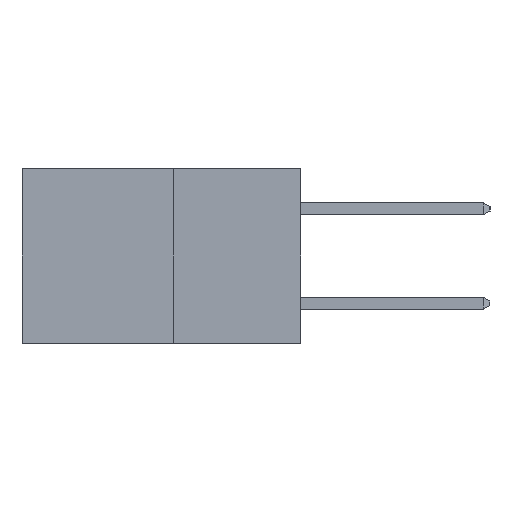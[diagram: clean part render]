
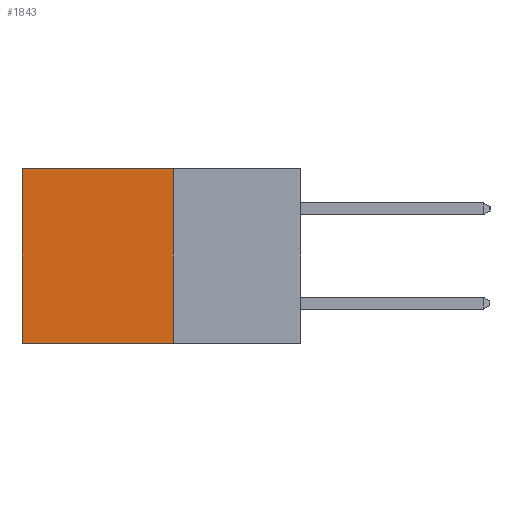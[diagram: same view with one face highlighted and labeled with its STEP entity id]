
A CAD part, left-side view. The second image highlights one B-rep face of the part: STEP entity #1843.
In plain terms, the highlighted planar face has unit normal (-1, 0, 0).
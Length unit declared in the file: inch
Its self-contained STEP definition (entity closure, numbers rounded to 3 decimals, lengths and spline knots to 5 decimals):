
#113 = ORIENTED_EDGE ( 'NONE', *, *, #7883, .F. ) ;
#327 = VERTEX_POINT ( 'NONE', #982 ) ;
#608 = CARTESIAN_POINT ( 'NONE',  ( 0.277, 0.27, 0. ) ) ;
#847 = ORIENTED_EDGE ( 'NONE', *, *, #9786, .T. ) ;
#982 = CARTESIAN_POINT ( 'NONE',  ( 0.277, 0.59, -0.37 ) ) ;
#1668 = AXIS2_PLACEMENT_3D ( 'NONE', #6906, #10502, #9858 ) ;
#1713 = DIRECTION ( 'NONE',  ( 0., 0., -1. ) ) ;
#1843 = ADVANCED_FACE ( 'NONE', ( #11647 ), #8633, .F. ) ;
#1958 = VECTOR ( 'NONE', #9533, 39.37008 ) ;
#2828 = CARTESIAN_POINT ( 'NONE',  ( 0.277, 0.27, -0.37 ) ) ;
#2880 = CARTESIAN_POINT ( 'NONE',  ( 0.277, 0.27, -0.37 ) ) ;
#4677 = DIRECTION ( 'NONE',  ( 0., 1., 0. ) ) ;
#4868 = LINE ( 'NONE', #8497, #1958 ) ;
#6008 = EDGE_CURVE ( 'NONE', #12313, #327, #11225, .T. ) ;
#6906 = CARTESIAN_POINT ( 'NONE',  ( 0.277, 0.27, -0.37 ) ) ;
#7883 = EDGE_CURVE ( 'NONE', #11270, #327, #4868, .T. ) ;
#8324 = ORIENTED_EDGE ( 'NONE', *, *, #6008, .T. ) ;
#8455 = VECTOR ( 'NONE', #12710, 39.37008 ) ;
#8497 = CARTESIAN_POINT ( 'NONE',  ( 0.277, 0.27, -0.37 ) ) ;
#8633 = PLANE ( 'NONE',  #1668 ) ;
#9533 = DIRECTION ( 'NONE',  ( 0., 1., 0. ) ) ;
#9584 = CARTESIAN_POINT ( 'NONE',  ( 0.277, 0.59, 0. ) ) ;
#9606 = VECTOR ( 'NONE', #1713, 39.37008 ) ;
#9786 = EDGE_CURVE ( 'NONE', #12674, #12313, #10773, .T. ) ;
#9858 = DIRECTION ( 'NONE',  ( 0., 0., -1. ) ) ;
#10502 = DIRECTION ( 'NONE',  ( 1., 0., 0. ) ) ;
#10773 = LINE ( 'NONE', #10856, #11122 ) ;
#10856 = CARTESIAN_POINT ( 'NONE',  ( 0.277, 0.27, 0. ) ) ;
#11122 = VECTOR ( 'NONE', #4677, 39.37008 ) ;
#11225 = LINE ( 'NONE', #11667, #8455 ) ;
#11249 = EDGE_CURVE ( 'NONE', #12674, #11270, #12746, .T. ) ;
#11270 = VERTEX_POINT ( 'NONE', #2880 ) ;
#11439 = ORIENTED_EDGE ( 'NONE', *, *, #11249, .F. ) ;
#11647 = FACE_OUTER_BOUND ( 'NONE', #12697, .T. ) ;
#11667 = CARTESIAN_POINT ( 'NONE',  ( 0.277, 0.59, -0.37 ) ) ;
#12313 = VERTEX_POINT ( 'NONE', #9584 ) ;
#12674 = VERTEX_POINT ( 'NONE', #608 ) ;
#12697 = EDGE_LOOP ( 'NONE', ( #8324, #113, #11439, #847 ) ) ;
#12710 = DIRECTION ( 'NONE',  ( 0., 0., -1. ) ) ;
#12746 = LINE ( 'NONE', #2828, #9606 ) ;
